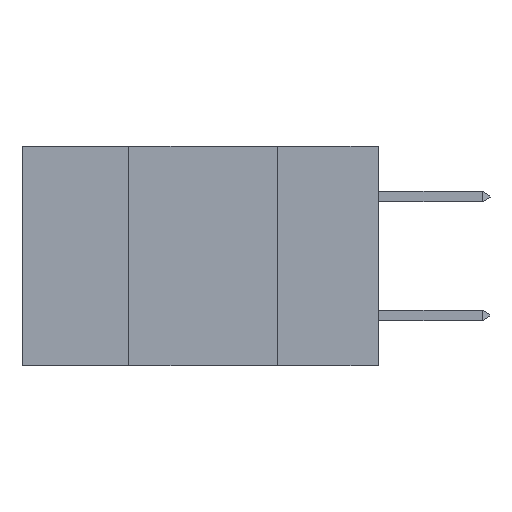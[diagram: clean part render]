
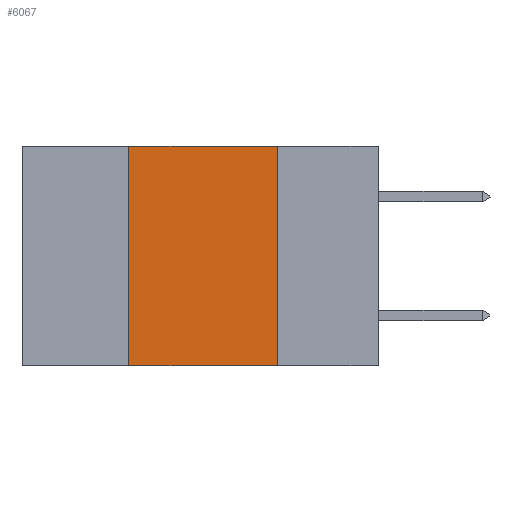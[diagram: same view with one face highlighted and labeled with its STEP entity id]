
A CAD part, left-side view. The second image highlights one B-rep face of the part: STEP entity #6067.
In plain terms, the highlighted planar face has unit normal (-1, 0, 0).
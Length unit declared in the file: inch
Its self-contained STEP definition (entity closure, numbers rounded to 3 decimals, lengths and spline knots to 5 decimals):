
#540 = CARTESIAN_POINT ( 'NONE',  ( 0., 0.6, 0. ) ) ;
#585 = VERTEX_POINT ( 'NONE', #20430 ) ;
#678 = DIRECTION ( 'NONE',  ( 0., -1., 0. ) ) ;
#696 = VECTOR ( 'NONE', #21934, 39.37008 ) ;
#1102 = LINE ( 'NONE', #6195, #14825 ) ;
#1827 = ORIENTED_EDGE ( 'NONE', *, *, #15070, .F. ) ;
#2557 = ORIENTED_EDGE ( 'NONE', *, *, #8382, .F. ) ;
#2662 = DIRECTION ( 'NONE',  ( 1., 0., 0. ) ) ;
#2790 = VERTEX_POINT ( 'NONE', #3246 ) ;
#3246 = CARTESIAN_POINT ( 'NONE',  ( 0., 0.17, -0.37 ) ) ;
#3701 = VECTOR ( 'NONE', #19082, 39.37008 ) ;
#5296 = CARTESIAN_POINT ( 'NONE',  ( 0., 0.42, 0. ) ) ;
#5401 = CARTESIAN_POINT ( 'NONE',  ( 0., 0.42, 0. ) ) ;
#6067 = ADVANCED_FACE ( 'NONE', ( #11410 ), #12954, .F. ) ;
#6195 = CARTESIAN_POINT ( 'NONE',  ( 0., 0.6, -0.37 ) ) ;
#7075 = DIRECTION ( 'NONE',  ( 0., 0., -1. ) ) ;
#7586 = ORIENTED_EDGE ( 'NONE', *, *, #13945, .F. ) ;
#8382 = EDGE_CURVE ( 'NONE', #11579, #585, #16592, .T. ) ;
#8487 = CARTESIAN_POINT ( 'NONE',  ( 0., 0.17, 0. ) ) ;
#9596 = CARTESIAN_POINT ( 'NONE',  ( 0., 0.42, -0.37 ) ) ;
#10988 = LINE ( 'NONE', #8487, #696 ) ;
#11410 = FACE_OUTER_BOUND ( 'NONE', #20759, .T. ) ;
#11579 = VERTEX_POINT ( 'NONE', #5401 ) ;
#12713 = VERTEX_POINT ( 'NONE', #9596 ) ;
#12796 = EDGE_CURVE ( 'NONE', #12713, #2790, #1102, .T. ) ;
#12925 = CARTESIAN_POINT ( 'NONE',  ( 0., 0.6, 0. ) ) ;
#12954 = PLANE ( 'NONE',  #17545 ) ;
#13945 = EDGE_CURVE ( 'NONE', #12713, #11579, #17122, .T. ) ;
#14825 = VECTOR ( 'NONE', #678, 39.37008 ) ;
#15070 = EDGE_CURVE ( 'NONE', #585, #2790, #10988, .T. ) ;
#16076 = VECTOR ( 'NONE', #18286, 39.37008 ) ;
#16592 = LINE ( 'NONE', #540, #16076 ) ;
#17122 = LINE ( 'NONE', #5296, #3701 ) ;
#17545 = AXIS2_PLACEMENT_3D ( 'NONE', #12925, #2662, #7075 ) ;
#18286 = DIRECTION ( 'NONE',  ( 0., -1., 0. ) ) ;
#19082 = DIRECTION ( 'NONE',  ( 0., 0., 1. ) ) ;
#20107 = ORIENTED_EDGE ( 'NONE', *, *, #12796, .T. ) ;
#20430 = CARTESIAN_POINT ( 'NONE',  ( 0., 0.17, 0. ) ) ;
#20759 = EDGE_LOOP ( 'NONE', ( #1827, #2557, #7586, #20107 ) ) ;
#21934 = DIRECTION ( 'NONE',  ( 0., 0., -1. ) ) ;
